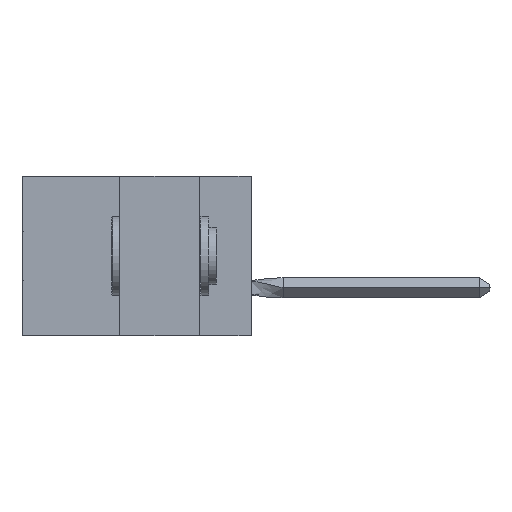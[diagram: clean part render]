
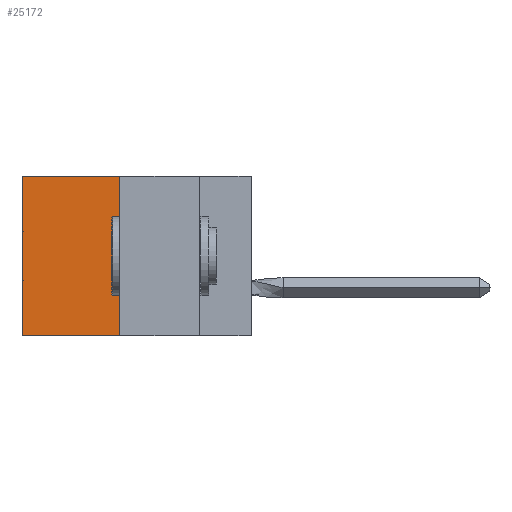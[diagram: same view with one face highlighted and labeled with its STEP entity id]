
A CAD part, left-side view. The second image highlights one B-rep face of the part: STEP entity #25172.
In plain terms, the highlighted planar face has unit normal (-1, 0, 0).
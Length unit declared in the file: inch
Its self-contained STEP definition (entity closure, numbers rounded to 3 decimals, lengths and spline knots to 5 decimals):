
#504 = LINE ( 'NONE', #30365, #26590 ) ;
#925 = DIRECTION ( 'NONE',  ( 1., 0., 0. ) ) ;
#1536 = VECTOR ( 'NONE', #23930, 39.37008 ) ;
#4338 = DIRECTION ( 'NONE',  ( 0., 1., 0. ) ) ;
#4449 = VERTEX_POINT ( 'NONE', #7687 ) ;
#4844 = EDGE_CURVE ( 'NONE', #36110, #13263, #504, .T. ) ;
#4850 = EDGE_CURVE ( 'NONE', #4449, #36110, #15894, .T. ) ;
#5085 = VECTOR ( 'NONE', #25050, 39.37008 ) ;
#6927 = AXIS2_PLACEMENT_3D ( 'NONE', #40161, #925, #10818 ) ;
#7687 = CARTESIAN_POINT ( 'NONE',  ( 0.305, 0.413, 0. ) ) ;
#10506 = PLANE ( 'NONE',  #6927 ) ;
#10818 = DIRECTION ( 'NONE',  ( 0., 0., -1. ) ) ;
#11491 = CARTESIAN_POINT ( 'NONE',  ( 0.305, 0.413, 0. ) ) ;
#13263 = VERTEX_POINT ( 'NONE', #33061 ) ;
#13770 = LINE ( 'NONE', #34898, #5085 ) ;
#14917 = ORIENTED_EDGE ( 'NONE', *, *, #31680, .T. ) ;
#15894 = LINE ( 'NONE', #36501, #1536 ) ;
#16172 = LINE ( 'NONE', #11491, #33058 ) ;
#21453 = CARTESIAN_POINT ( 'NONE',  ( 0.305, 0.72, 0. ) ) ;
#22981 = EDGE_CURVE ( 'NONE', #4449, #23949, #16172, .T. ) ;
#23930 = DIRECTION ( 'NONE',  ( 0., 0., -1. ) ) ;
#23949 = VERTEX_POINT ( 'NONE', #21453 ) ;
#24849 = ORIENTED_EDGE ( 'NONE', *, *, #4850, .F. ) ;
#24919 = FACE_OUTER_BOUND ( 'NONE', #30334, .T. ) ;
#25050 = DIRECTION ( 'NONE',  ( 0., 0., -1. ) ) ;
#25172 = ADVANCED_FACE ( 'NONE', ( #24919 ), #10506, .F. ) ;
#26590 = VECTOR ( 'NONE', #4338, 39.37008 ) ;
#26724 = DIRECTION ( 'NONE',  ( 0., 1., 0. ) ) ;
#30334 = EDGE_LOOP ( 'NONE', ( #14917, #39890, #24849, #34250 ) ) ;
#30365 = CARTESIAN_POINT ( 'NONE',  ( 0.305, 0.413, -0.5 ) ) ;
#30436 = CARTESIAN_POINT ( 'NONE',  ( 0.305, 0.413, -0.5 ) ) ;
#31680 = EDGE_CURVE ( 'NONE', #23949, #13263, #13770, .T. ) ;
#33058 = VECTOR ( 'NONE', #26724, 39.37008 ) ;
#33061 = CARTESIAN_POINT ( 'NONE',  ( 0.305, 0.72, -0.5 ) ) ;
#34250 = ORIENTED_EDGE ( 'NONE', *, *, #22981, .T. ) ;
#34898 = CARTESIAN_POINT ( 'NONE',  ( 0.305, 0.72, -0.5 ) ) ;
#36110 = VERTEX_POINT ( 'NONE', #30436 ) ;
#36501 = CARTESIAN_POINT ( 'NONE',  ( 0.305, 0.413, -0.5 ) ) ;
#39890 = ORIENTED_EDGE ( 'NONE', *, *, #4844, .F. ) ;
#40161 = CARTESIAN_POINT ( 'NONE',  ( 0.305, 0.413, -0.5 ) ) ;
